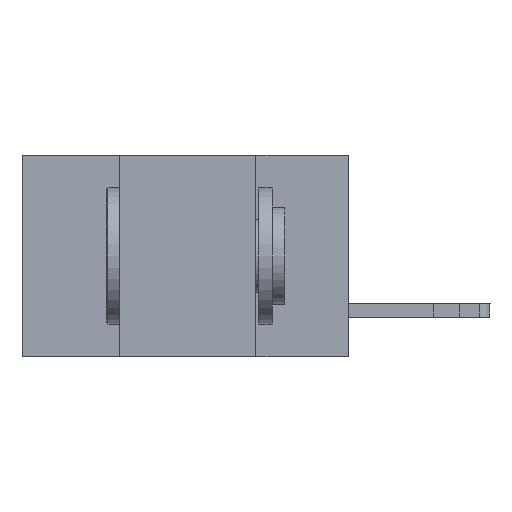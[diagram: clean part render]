
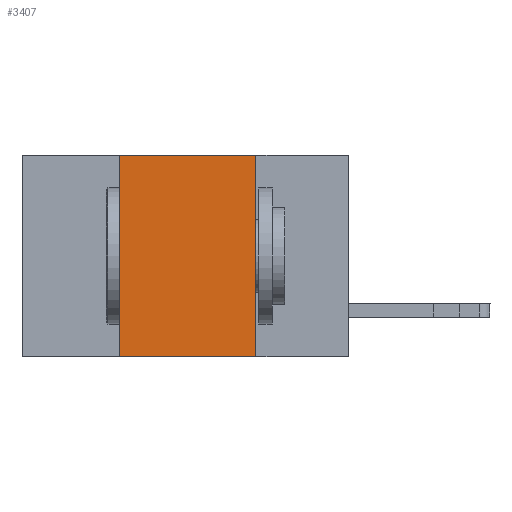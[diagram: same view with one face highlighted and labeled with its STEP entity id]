
A CAD part, left-side view. The second image highlights one B-rep face of the part: STEP entity #3407.
In plain terms, the highlighted planar face has unit normal (-1, 0, 0).
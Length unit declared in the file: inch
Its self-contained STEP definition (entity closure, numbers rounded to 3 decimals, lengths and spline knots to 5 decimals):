
#36 = LINE ( 'NONE', #11453, #12478 ) ;
#711 = DIRECTION ( 'NONE',  ( 0., -1., 0. ) ) ;
#1020 = PLANE ( 'NONE',  #12186 ) ;
#2050 = VERTEX_POINT ( 'NONE', #4602 ) ;
#2227 = CARTESIAN_POINT ( 'NONE',  ( 0., 0.42, 0. ) ) ;
#2855 = VECTOR ( 'NONE', #711, 39.37008 ) ;
#3170 = EDGE_CURVE ( 'NONE', #2050, #4778, #5989, .T. ) ;
#3407 = ADVANCED_FACE ( 'NONE', ( #14632 ), #1020, .F. ) ;
#3498 = CARTESIAN_POINT ( 'NONE',  ( 0., 0.42, -0.37 ) ) ;
#3652 = DIRECTION ( 'NONE',  ( 0., 0., -1. ) ) ;
#4450 = EDGE_CURVE ( 'NONE', #5233, #12595, #13950, .T. ) ;
#4602 = CARTESIAN_POINT ( 'NONE',  ( 0., 0.42, -0.37 ) ) ;
#4778 = VERTEX_POINT ( 'NONE', #2227 ) ;
#5233 = VERTEX_POINT ( 'NONE', #11010 ) ;
#5255 = EDGE_CURVE ( 'NONE', #4778, #5233, #7852, .T. ) ;
#5515 = CARTESIAN_POINT ( 'NONE',  ( 0., 0.6, 0. ) ) ;
#5533 = CARTESIAN_POINT ( 'NONE',  ( 0., 0.6, 0. ) ) ;
#5844 = CARTESIAN_POINT ( 'NONE',  ( 0., 0.17, -0.37 ) ) ;
#5989 = LINE ( 'NONE', #3498, #7389 ) ;
#6725 = ORIENTED_EDGE ( 'NONE', *, *, #10113, .T. ) ;
#6749 = CARTESIAN_POINT ( 'NONE',  ( 0., 0.17, -0.37 ) ) ;
#6800 = DIRECTION ( 'NONE',  ( 0., -1., 0. ) ) ;
#7357 = ORIENTED_EDGE ( 'NONE', *, *, #4450, .F. ) ;
#7389 = VECTOR ( 'NONE', #11557, 39.37008 ) ;
#7852 = LINE ( 'NONE', #5515, #2855 ) ;
#10113 = EDGE_CURVE ( 'NONE', #2050, #12595, #36, .T. ) ;
#10285 = VECTOR ( 'NONE', #3652, 39.37008 ) ;
#11010 = CARTESIAN_POINT ( 'NONE',  ( 0., 0.17, 0. ) ) ;
#11453 = CARTESIAN_POINT ( 'NONE',  ( 0., 0.6, -0.37 ) ) ;
#11557 = DIRECTION ( 'NONE',  ( 0., 0., 1. ) ) ;
#12186 = AXIS2_PLACEMENT_3D ( 'NONE', #5533, #14479, #13438 ) ;
#12336 = ORIENTED_EDGE ( 'NONE', *, *, #3170, .F. ) ;
#12478 = VECTOR ( 'NONE', #6800, 39.37008 ) ;
#12568 = EDGE_LOOP ( 'NONE', ( #7357, #14580, #12336, #6725 ) ) ;
#12595 = VERTEX_POINT ( 'NONE', #6749 ) ;
#13438 = DIRECTION ( 'NONE',  ( 0., 0., -1. ) ) ;
#13950 = LINE ( 'NONE', #5844, #10285 ) ;
#14479 = DIRECTION ( 'NONE',  ( 1., 0., 0. ) ) ;
#14580 = ORIENTED_EDGE ( 'NONE', *, *, #5255, .F. ) ;
#14632 = FACE_OUTER_BOUND ( 'NONE', #12568, .T. ) ;
